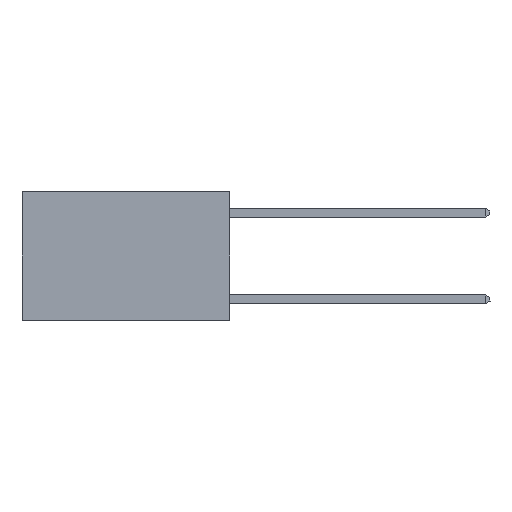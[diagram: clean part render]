
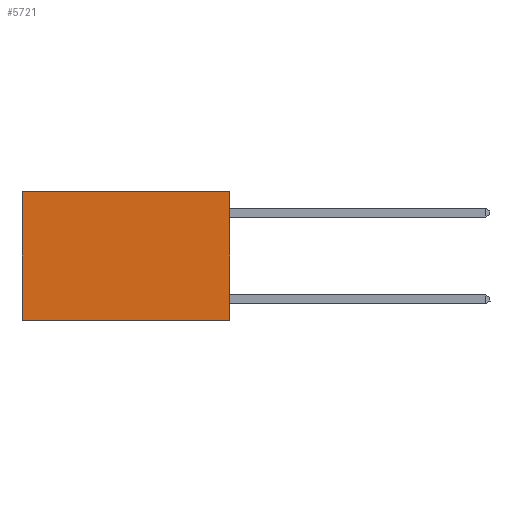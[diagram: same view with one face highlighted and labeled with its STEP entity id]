
A CAD part, left-side view. The second image highlights one B-rep face of the part: STEP entity #5721.
In plain terms, the highlighted planar face has unit normal (-1, 0, 0).
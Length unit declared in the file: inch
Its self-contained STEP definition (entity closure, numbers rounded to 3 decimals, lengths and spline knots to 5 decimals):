
#177 = ORIENTED_EDGE ( 'NONE', *, *, #11310, .T. ) ;
#992 = VERTEX_POINT ( 'NONE', #7490 ) ;
#1141 = CARTESIAN_POINT ( 'NONE',  ( 0.2625, 0., 0. ) ) ;
#2147 = VERTEX_POINT ( 'NONE', #8052 ) ;
#2331 = PLANE ( 'NONE',  #7030 ) ;
#2720 = DIRECTION ( 'NONE',  ( 0., 0., -1. ) ) ;
#3413 = VERTEX_POINT ( 'NONE', #17372 ) ;
#3496 = LINE ( 'NONE', #17964, #15270 ) ;
#4141 = ORIENTED_EDGE ( 'NONE', *, *, #14205, .T. ) ;
#4234 = VECTOR ( 'NONE', #2720, 39.37008 ) ;
#4285 = VECTOR ( 'NONE', #10278, 39.37008 ) ;
#5457 = DIRECTION ( 'NONE',  ( 0., 0., -1. ) ) ;
#5721 = ADVANCED_FACE ( 'NONE', ( #19081 ), #2331, .F. ) ;
#6538 = EDGE_CURVE ( 'NONE', #992, #3413, #16933, .T. ) ;
#7030 = AXIS2_PLACEMENT_3D ( 'NONE', #13097, #14607, #5457 ) ;
#7061 = VECTOR ( 'NONE', #13500, 39.37008 ) ;
#7490 = CARTESIAN_POINT ( 'NONE',  ( 0.2625, 0., 0. ) ) ;
#7869 = LINE ( 'NONE', #17860, #4285 ) ;
#8052 = CARTESIAN_POINT ( 'NONE',  ( 0.2625, 0.6, -0.37 ) ) ;
#10278 = DIRECTION ( 'NONE',  ( 0., 0., -1. ) ) ;
#10444 = CARTESIAN_POINT ( 'NONE',  ( 0.2625, 0., 0. ) ) ;
#10885 = ORIENTED_EDGE ( 'NONE', *, *, #12716, .F. ) ;
#11157 = LINE ( 'NONE', #10444, #7061 ) ;
#11310 = EDGE_CURVE ( 'NONE', #14180, #2147, #7869, .T. ) ;
#12716 = EDGE_CURVE ( 'NONE', #3413, #2147, #3496, .T. ) ;
#13097 = CARTESIAN_POINT ( 'NONE',  ( 0.2625, 0., 0. ) ) ;
#13500 = DIRECTION ( 'NONE',  ( 0., 1., 0. ) ) ;
#14180 = VERTEX_POINT ( 'NONE', #18023 ) ;
#14205 = EDGE_CURVE ( 'NONE', #992, #14180, #11157, .T. ) ;
#14607 = DIRECTION ( 'NONE',  ( 1., 0., 0. ) ) ;
#14970 = EDGE_LOOP ( 'NONE', ( #177, #10885, #19438, #4141 ) ) ;
#14981 = DIRECTION ( 'NONE',  ( 0., 1., 0. ) ) ;
#15270 = VECTOR ( 'NONE', #14981, 39.37008 ) ;
#16933 = LINE ( 'NONE', #1141, #4234 ) ;
#17372 = CARTESIAN_POINT ( 'NONE',  ( 0.2625, 0., -0.37 ) ) ;
#17860 = CARTESIAN_POINT ( 'NONE',  ( 0.2625, 0.6, 0. ) ) ;
#17964 = CARTESIAN_POINT ( 'NONE',  ( 0.2625, 0., -0.37 ) ) ;
#18023 = CARTESIAN_POINT ( 'NONE',  ( 0.2625, 0.6, 0. ) ) ;
#19081 = FACE_OUTER_BOUND ( 'NONE', #14970, .T. ) ;
#19438 = ORIENTED_EDGE ( 'NONE', *, *, #6538, .F. ) ;
